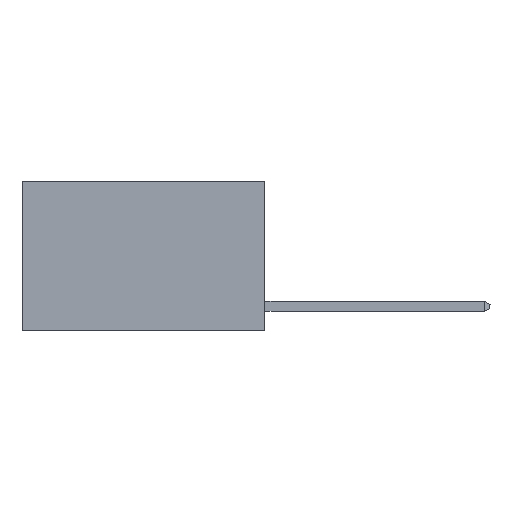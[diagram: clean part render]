
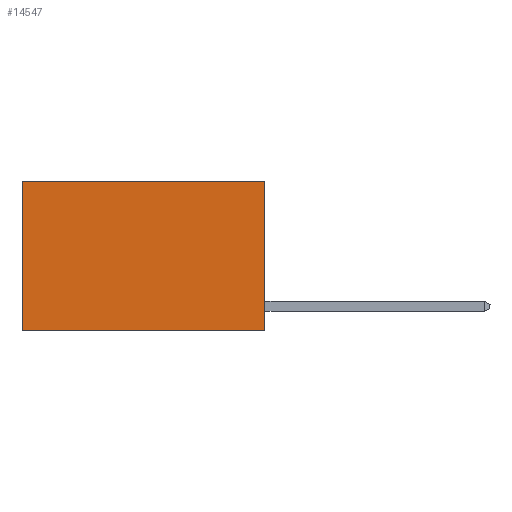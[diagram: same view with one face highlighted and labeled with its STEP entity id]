
A CAD part, left-side view. The second image highlights one B-rep face of the part: STEP entity #14547.
In plain terms, the highlighted planar face has unit normal (-1, 0, 0).
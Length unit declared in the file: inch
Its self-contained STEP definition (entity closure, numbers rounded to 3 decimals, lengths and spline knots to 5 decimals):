
#828 = VECTOR ( 'NONE', #13562, 39.37008 ) ;
#1047 = ORIENTED_EDGE ( 'NONE', *, *, #3867, .F. ) ;
#3867 = EDGE_CURVE ( 'NONE', #10806, #9447, #7168, .T. ) ;
#4352 = CARTESIAN_POINT ( 'NONE',  ( 0.2625, 0., 0. ) ) ;
#5162 = LINE ( 'NONE', #8034, #14008 ) ;
#6219 = CARTESIAN_POINT ( 'NONE',  ( 0.2625, 0.6, 0. ) ) ;
#7081 = LINE ( 'NONE', #4352, #11356 ) ;
#7168 = LINE ( 'NONE', #9934, #10219 ) ;
#7238 = FACE_OUTER_BOUND ( 'NONE', #18443, .T. ) ;
#8034 = CARTESIAN_POINT ( 'NONE',  ( 0.2625, 0., -0.37 ) ) ;
#8780 = VERTEX_POINT ( 'NONE', #16887 ) ;
#8869 = EDGE_CURVE ( 'NONE', #9447, #8780, #5162, .T. ) ;
#8966 = LINE ( 'NONE', #6219, #828 ) ;
#9127 = EDGE_CURVE ( 'NONE', #14012, #8780, #8966, .T. ) ;
#9447 = VERTEX_POINT ( 'NONE', #12810 ) ;
#9934 = CARTESIAN_POINT ( 'NONE',  ( 0.2625, 0., 0. ) ) ;
#10219 = VECTOR ( 'NONE', #18796, 39.37008 ) ;
#10806 = VERTEX_POINT ( 'NONE', #17158 ) ;
#11356 = VECTOR ( 'NONE', #15994, 39.37008 ) ;
#11712 = DIRECTION ( 'NONE',  ( 1., 0., 0. ) ) ;
#12730 = CARTESIAN_POINT ( 'NONE',  ( 0.2625, 0.6, 0. ) ) ;
#12810 = CARTESIAN_POINT ( 'NONE',  ( 0.2625, 0., -0.37 ) ) ;
#12851 = EDGE_CURVE ( 'NONE', #10806, #14012, #7081, .T. ) ;
#13255 = CARTESIAN_POINT ( 'NONE',  ( 0.2625, 0., 0. ) ) ;
#13562 = DIRECTION ( 'NONE',  ( 0., 0., -1. ) ) ;
#14008 = VECTOR ( 'NONE', #15631, 39.37008 ) ;
#14012 = VERTEX_POINT ( 'NONE', #12730 ) ;
#14547 = ADVANCED_FACE ( 'NONE', ( #7238 ), #16162, .F. ) ;
#15120 = ORIENTED_EDGE ( 'NONE', *, *, #9127, .T. ) ;
#15631 = DIRECTION ( 'NONE',  ( 0., 1., 0. ) ) ;
#15923 = ORIENTED_EDGE ( 'NONE', *, *, #8869, .F. ) ;
#15994 = DIRECTION ( 'NONE',  ( 0., 1., 0. ) ) ;
#16162 = PLANE ( 'NONE',  #18489 ) ;
#16322 = ORIENTED_EDGE ( 'NONE', *, *, #12851, .T. ) ;
#16887 = CARTESIAN_POINT ( 'NONE',  ( 0.2625, 0.6, -0.37 ) ) ;
#17158 = CARTESIAN_POINT ( 'NONE',  ( 0.2625, 0., 0. ) ) ;
#18443 = EDGE_LOOP ( 'NONE', ( #15120, #15923, #1047, #16322 ) ) ;
#18489 = AXIS2_PLACEMENT_3D ( 'NONE', #13255, #11712, #18957 ) ;
#18796 = DIRECTION ( 'NONE',  ( 0., 0., -1. ) ) ;
#18957 = DIRECTION ( 'NONE',  ( 0., 0., -1. ) ) ;
